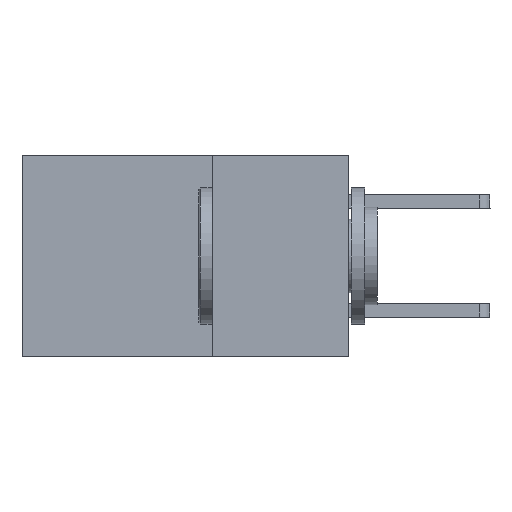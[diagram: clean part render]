
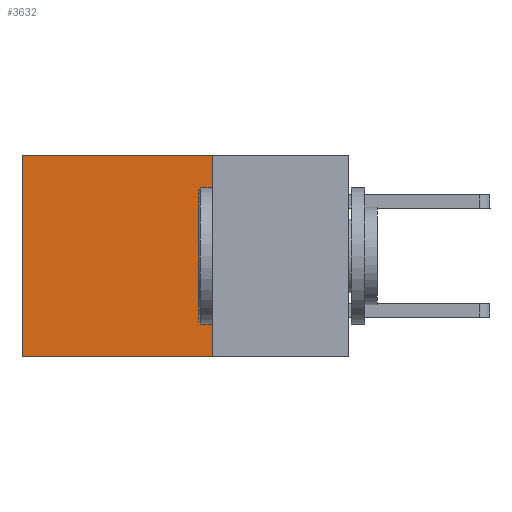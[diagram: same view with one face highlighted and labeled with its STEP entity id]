
A CAD part, left-side view. The second image highlights one B-rep face of the part: STEP entity #3632.
In plain terms, the highlighted planar face has unit normal (-1, 0, 0).
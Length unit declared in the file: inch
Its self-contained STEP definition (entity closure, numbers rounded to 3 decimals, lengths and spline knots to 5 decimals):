
#464 = VERTEX_POINT ( 'NONE', #3098 ) ;
#845 = DIRECTION ( 'NONE',  ( 0., 1., 0. ) ) ;
#1380 = VECTOR ( 'NONE', #6754, 39.37008 ) ;
#1522 = CARTESIAN_POINT ( 'NONE',  ( 0.2615, 0.25, 0. ) ) ;
#1607 = FACE_OUTER_BOUND ( 'NONE', #1752, .T. ) ;
#1657 = EDGE_CURVE ( 'NONE', #8096, #1693, #5034, .T. ) ;
#1662 = DIRECTION ( 'NONE',  ( 1., 0., 0. ) ) ;
#1679 = VECTOR ( 'NONE', #3789, 39.37008 ) ;
#1693 = VERTEX_POINT ( 'NONE', #3628 ) ;
#1752 = EDGE_LOOP ( 'NONE', ( #6083, #6739, #3260, #3146 ) ) ;
#1842 = DIRECTION ( 'NONE',  ( 0., 0., -1. ) ) ;
#2556 = VERTEX_POINT ( 'NONE', #5243 ) ;
#2622 = LINE ( 'NONE', #6128, #3831 ) ;
#3082 = PLANE ( 'NONE',  #6186 ) ;
#3098 = CARTESIAN_POINT ( 'NONE',  ( 0.2615, 0.25, -0.37 ) ) ;
#3146 = ORIENTED_EDGE ( 'NONE', *, *, #1657, .T. ) ;
#3228 = CARTESIAN_POINT ( 'NONE',  ( 0.2615, 0.25, -0.37 ) ) ;
#3260 = ORIENTED_EDGE ( 'NONE', *, *, #7926, .F. ) ;
#3628 = CARTESIAN_POINT ( 'NONE',  ( 0.2615, 0.6, 0. ) ) ;
#3632 = ADVANCED_FACE ( 'NONE', ( #1607 ), #3082, .F. ) ;
#3777 = DIRECTION ( 'NONE',  ( 0., 0., -1. ) ) ;
#3789 = DIRECTION ( 'NONE',  ( 0., 1., 0. ) ) ;
#3831 = VECTOR ( 'NONE', #1842, 39.37008 ) ;
#3882 = LINE ( 'NONE', #3228, #1679 ) ;
#4252 = EDGE_CURVE ( 'NONE', #464, #2556, #3882, .T. ) ;
#4275 = EDGE_CURVE ( 'NONE', #1693, #2556, #8810, .T. ) ;
#4416 = CARTESIAN_POINT ( 'NONE',  ( 0.2615, 0.25, -0.37 ) ) ;
#4592 = VECTOR ( 'NONE', #845, 39.37008 ) ;
#5034 = LINE ( 'NONE', #1522, #4592 ) ;
#5243 = CARTESIAN_POINT ( 'NONE',  ( 0.2615, 0.6, -0.37 ) ) ;
#5699 = CARTESIAN_POINT ( 'NONE',  ( 0.2615, 0.25, 0. ) ) ;
#6083 = ORIENTED_EDGE ( 'NONE', *, *, #4275, .T. ) ;
#6128 = CARTESIAN_POINT ( 'NONE',  ( 0.2615, 0.25, -0.37 ) ) ;
#6186 = AXIS2_PLACEMENT_3D ( 'NONE', #4416, #1662, #3777 ) ;
#6739 = ORIENTED_EDGE ( 'NONE', *, *, #4252, .F. ) ;
#6754 = DIRECTION ( 'NONE',  ( 0., 0., -1. ) ) ;
#7926 = EDGE_CURVE ( 'NONE', #8096, #464, #2622, .T. ) ;
#8092 = CARTESIAN_POINT ( 'NONE',  ( 0.2615, 0.6, -0.37 ) ) ;
#8096 = VERTEX_POINT ( 'NONE', #5699 ) ;
#8810 = LINE ( 'NONE', #8092, #1380 ) ;
